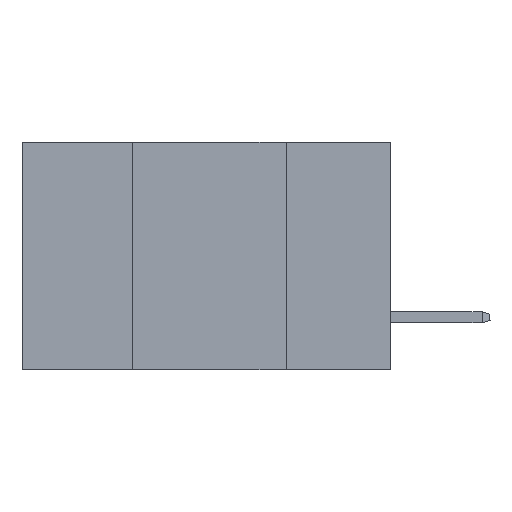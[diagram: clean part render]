
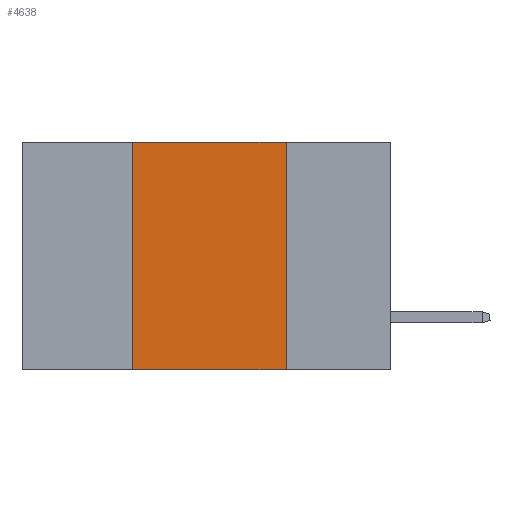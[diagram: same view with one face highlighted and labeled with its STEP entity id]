
A CAD part, left-side view. The second image highlights one B-rep face of the part: STEP entity #4638.
In plain terms, the highlighted planar face has unit normal (-1, 0, 0).
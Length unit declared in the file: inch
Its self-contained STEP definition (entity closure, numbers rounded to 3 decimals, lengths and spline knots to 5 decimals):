
#156 = DIRECTION ( 'NONE',  ( 0., -1., 0. ) ) ;
#158 = LINE ( 'NONE', #4593, #17810 ) ;
#2193 = VECTOR ( 'NONE', #156, 39.37008 ) ;
#3099 = CARTESIAN_POINT ( 'NONE',  ( 0., 0.6, 0. ) ) ;
#3979 = CARTESIAN_POINT ( 'NONE',  ( 0., 0.6, 0. ) ) ;
#4149 = VECTOR ( 'NONE', #18485, 39.37008 ) ;
#4593 = CARTESIAN_POINT ( 'NONE',  ( 0., 0.42, 0. ) ) ;
#4638 = ADVANCED_FACE ( 'NONE', ( #11205 ), #11216, .F. ) ;
#5328 = EDGE_CURVE ( 'NONE', #12259, #19466, #9047, .T. ) ;
#5926 = DIRECTION ( 'NONE',  ( 0., 0., -1. ) ) ;
#5987 = VERTEX_POINT ( 'NONE', #17700 ) ;
#6032 = AXIS2_PLACEMENT_3D ( 'NONE', #3979, #14499, #17430 ) ;
#6459 = VECTOR ( 'NONE', #5926, 39.37008 ) ;
#7042 = ORIENTED_EDGE ( 'NONE', *, *, #5328, .F. ) ;
#9047 = LINE ( 'NONE', #16606, #6459 ) ;
#9081 = EDGE_CURVE ( 'NONE', #18185, #5987, #158, .T. ) ;
#9512 = EDGE_CURVE ( 'NONE', #18185, #19466, #13079, .T. ) ;
#10220 = LINE ( 'NONE', #3099, #2193 ) ;
#10616 = CARTESIAN_POINT ( 'NONE',  ( 0., 0.42, -0.37 ) ) ;
#10996 = EDGE_CURVE ( 'NONE', #5987, #12259, #10220, .T. ) ;
#11205 = FACE_OUTER_BOUND ( 'NONE', #16838, .T. ) ;
#11216 = PLANE ( 'NONE',  #6032 ) ;
#11300 = CARTESIAN_POINT ( 'NONE',  ( 0., 0.6, -0.37 ) ) ;
#11456 = CARTESIAN_POINT ( 'NONE',  ( 0., 0.17, 0. ) ) ;
#12229 = ORIENTED_EDGE ( 'NONE', *, *, #10996, .F. ) ;
#12259 = VERTEX_POINT ( 'NONE', #11456 ) ;
#13079 = LINE ( 'NONE', #11300, #4149 ) ;
#14499 = DIRECTION ( 'NONE',  ( 1., 0., 0. ) ) ;
#15331 = ORIENTED_EDGE ( 'NONE', *, *, #9512, .T. ) ;
#16586 = DIRECTION ( 'NONE',  ( 0., 0., 1. ) ) ;
#16606 = CARTESIAN_POINT ( 'NONE',  ( 0., 0.17, 0. ) ) ;
#16838 = EDGE_LOOP ( 'NONE', ( #7042, #12229, #19138, #15331 ) ) ;
#17430 = DIRECTION ( 'NONE',  ( 0., 0., -1. ) ) ;
#17533 = CARTESIAN_POINT ( 'NONE',  ( 0., 0.17, -0.37 ) ) ;
#17700 = CARTESIAN_POINT ( 'NONE',  ( 0., 0.42, 0. ) ) ;
#17810 = VECTOR ( 'NONE', #16586, 39.37008 ) ;
#18185 = VERTEX_POINT ( 'NONE', #10616 ) ;
#18485 = DIRECTION ( 'NONE',  ( 0., -1., 0. ) ) ;
#19138 = ORIENTED_EDGE ( 'NONE', *, *, #9081, .F. ) ;
#19466 = VERTEX_POINT ( 'NONE', #17533 ) ;
